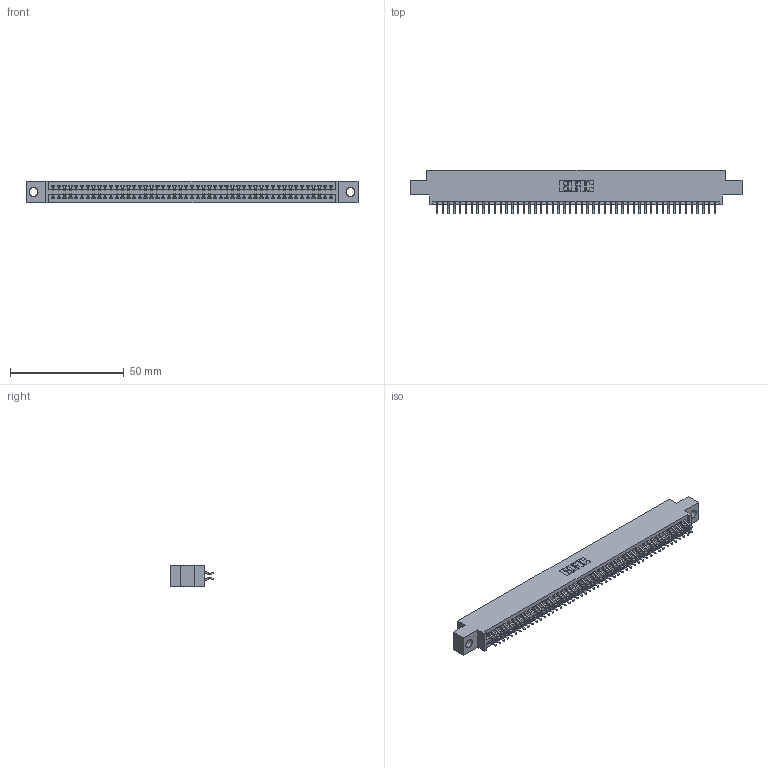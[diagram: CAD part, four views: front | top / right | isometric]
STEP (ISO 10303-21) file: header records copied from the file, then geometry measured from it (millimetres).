
FILE_DESCRIPTION (( 'STEP AP203' ), '1' );
FILE_NAME ('345-098-556-804.STEP', '2021-05-20T18:15:41', ( '' ), ( '' ), 'SwSTEP 2.0', 'SolidWorks 2020', '' );
FILE_SCHEMA (( 'CONFIG_CONTROL_DESIGN' ));
Length unit declared in the file: inch
Products named in the file (3): 345-292-001_556 Tail; 345-098-556-804; 345 Part_0.170 Offset - 0.156 Dia-TI
Assembly tree (99 placements, depth 2):
  345-098-556-804
    345 Part_0.170 Offset - 0.156 Dia-TI
    345-292-001_556 Tail  x98
Bounding box: 145.67 x 19.24 x 9.4 mm (x, y, z)
Volume: 13992.2 mm3; surface area: 20727.7 mm2
Topology: 99 solids, 99 shells, 5632 faces, 16755 edges, 11038 vertices
Faces by surface type: plane 3724, cylinder 1908
Entity records: 38275 total; most frequent: CARTESIAN_POINT 6430, ORIENTED_EDGE 6350, DIRECTION 5647, EDGE_CURVE 3175, VECTOR 2839, LINE 2839, VERTEX_POINT 2114, AXIS2_PLACEMENT_3D 1404
